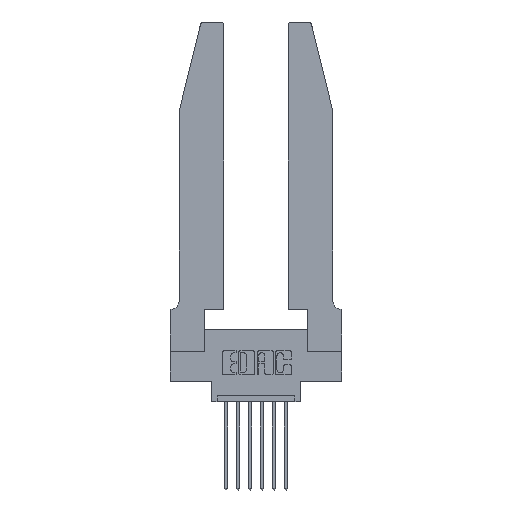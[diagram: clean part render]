
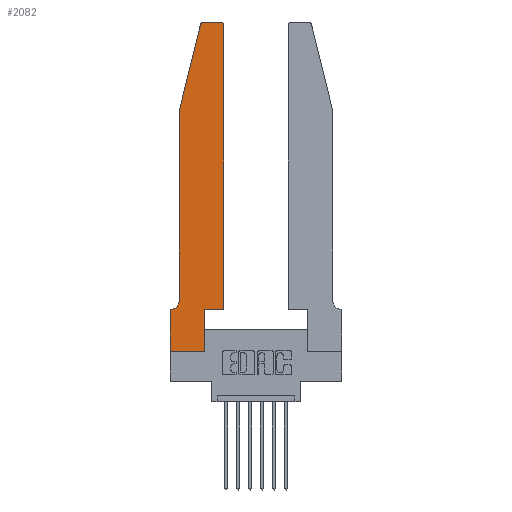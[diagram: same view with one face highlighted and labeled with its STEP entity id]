
A CAD part, top view. The second image highlights one B-rep face of the part: STEP entity #2082.
In plain terms, the highlighted planar face has unit normal (0, 0, 1).
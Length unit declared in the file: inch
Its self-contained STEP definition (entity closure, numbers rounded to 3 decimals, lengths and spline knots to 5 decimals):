
#66 = VECTOR ( 'NONE', #14003, 39.37008 ) ;
#102 = VECTOR ( 'NONE', #5840, 39.37008 ) ;
#453 = CARTESIAN_POINT ( 'NONE',  ( 0.4505, 0.35, 0.37 ) ) ;
#550 = CARTESIAN_POINT ( 'NONE',  ( 0.4205, 2.72, 0.37 ) ) ;
#649 = CARTESIAN_POINT ( 'NONE',  ( 0.2865, 0.35, 0.37 ) ) ;
#678 = EDGE_CURVE ( 'NONE', #8250, #14021, #8763, .T. ) ;
#988 = VERTEX_POINT ( 'NONE', #13932 ) ;
#1011 = ORIENTED_EDGE ( 'NONE', *, *, #9448, .T. ) ;
#1093 = VECTOR ( 'NONE', #13650, 39.37008 ) ;
#1171 = FACE_OUTER_BOUND ( 'NONE', #6539, .T. ) ;
#1270 = VERTEX_POINT ( 'NONE', #453 ) ;
#1389 = CARTESIAN_POINT ( 'NONE',  ( 0.284, 2.75, 0.37 ) ) ;
#1478 = VECTOR ( 'NONE', #7660, 39.37008 ) ;
#1817 = VERTEX_POINT ( 'NONE', #1389 ) ;
#1842 = VERTEX_POINT ( 'NONE', #7890 ) ;
#1893 = ORIENTED_EDGE ( 'NONE', *, *, #9332, .T. ) ;
#1906 = CARTESIAN_POINT ( 'NONE',  ( 0.0755, 2., 0.37 ) ) ;
#1942 = ORIENTED_EDGE ( 'NONE', *, *, #11887, .T. ) ;
#2082 = ADVANCED_FACE ( 'NONE', ( #1171 ), #2833, .T. ) ;
#2570 = DIRECTION ( 'NONE',  ( 0., 0., 1. ) ) ;
#2833 = PLANE ( 'NONE',  #11426 ) ;
#2865 = VERTEX_POINT ( 'NONE', #6434 ) ;
#2966 = EDGE_CURVE ( 'NONE', #1817, #988, #8417, .T. ) ;
#2976 = DIRECTION ( 'NONE',  ( 0., 0., -1. ) ) ;
#3628 = LINE ( 'NONE', #13742, #13936 ) ;
#3701 = ORIENTED_EDGE ( 'NONE', *, *, #10732, .T. ) ;
#3813 = DIRECTION ( 'NONE',  ( 1., 0., 0. ) ) ;
#3830 = LINE ( 'NONE', #8768, #14129 ) ;
#4001 = ORIENTED_EDGE ( 'NONE', *, *, #5350, .T. ) ;
#4075 = DIRECTION ( 'NONE',  ( -1., 0., 0. ) ) ;
#4324 = DIRECTION ( 'NONE',  ( 0., -1., 0. ) ) ;
#4795 = ORIENTED_EDGE ( 'NONE', *, *, #6961, .T. ) ;
#4895 = CARTESIAN_POINT ( 'NONE',  ( 0.4505, 0.35, 0.37 ) ) ;
#5023 = EDGE_CURVE ( 'NONE', #1842, #1270, #12653, .T. ) ;
#5350 = EDGE_CURVE ( 'NONE', #13321, #1817, #8893, .T. ) ;
#5401 = ORIENTED_EDGE ( 'NONE', *, *, #2966, .T. ) ;
#5441 = VERTEX_POINT ( 'NONE', #9337 ) ;
#5596 = VERTEX_POINT ( 'NONE', #7854 ) ;
#5840 = DIRECTION ( 'NONE',  ( -1., 0., 0. ) ) ;
#5863 = VECTOR ( 'NONE', #7314, 39.37008 ) ;
#6434 = CARTESIAN_POINT ( 'NONE',  ( 0., 0.35, 0.37 ) ) ;
#6539 = EDGE_LOOP ( 'NONE', ( #4001, #5401, #1942, #6580, #11002, #10204, #3701, #7214, #1011, #8343, #4795, #1893 ) ) ;
#6580 = ORIENTED_EDGE ( 'NONE', *, *, #678, .T. ) ;
#6613 = DIRECTION ( 'NONE',  ( 0., 1., 0. ) ) ;
#6961 = EDGE_CURVE ( 'NONE', #1270, #5596, #3830, .T. ) ;
#7214 = ORIENTED_EDGE ( 'NONE', *, *, #7489, .T. ) ;
#7291 = AXIS2_PLACEMENT_3D ( 'NONE', #9358, #11533, #8386 ) ;
#7314 = DIRECTION ( 'NONE',  ( 0., 1., 0. ) ) ;
#7489 = EDGE_CURVE ( 'NONE', #5441, #11415, #3628, .T. ) ;
#7660 = DIRECTION ( 'NONE',  ( 0., -1., 0. ) ) ;
#7854 = CARTESIAN_POINT ( 'NONE',  ( 0.4505, 2.72, 0.37 ) ) ;
#7890 = CARTESIAN_POINT ( 'NONE',  ( 0.2865, 0.35, 0.37 ) ) ;
#7938 = CIRCLE ( 'NONE', #13310, 0.07 ) ;
#7983 = CARTESIAN_POINT ( 'NONE',  ( 0.4205, 2.75, 0.37 ) ) ;
#8250 = VERTEX_POINT ( 'NONE', #10523 ) ;
#8343 = ORIENTED_EDGE ( 'NONE', *, *, #5023, .T. ) ;
#8351 = EDGE_CURVE ( 'NONE', #14021, #10306, #7938, .T. ) ;
#8386 = DIRECTION ( 'NONE',  ( 1., 0., 0. ) ) ;
#8417 = CIRCLE ( 'NONE', #7291, 0.03 ) ;
#8763 = LINE ( 'NONE', #9825, #11310 ) ;
#8768 = CARTESIAN_POINT ( 'NONE',  ( 0.4505, 0.35, 0.37 ) ) ;
#8779 = LINE ( 'NONE', #14285, #1478 ) ;
#8893 = LINE ( 'NONE', #9677, #11265 ) ;
#9332 = EDGE_CURVE ( 'NONE', #5596, #13321, #12201, .T. ) ;
#9337 = CARTESIAN_POINT ( 'NONE',  ( 0., 0., 0.37 ) ) ;
#9358 = CARTESIAN_POINT ( 'NONE',  ( 0.284, 2.72, 0.37 ) ) ;
#9448 = EDGE_CURVE ( 'NONE', #11415, #1842, #13917, .T. ) ;
#9677 = CARTESIAN_POINT ( 'NONE',  ( 0.2605, 2.75, 0.37 ) ) ;
#9793 = LINE ( 'NONE', #13311, #102 ) ;
#9825 = CARTESIAN_POINT ( 'NONE',  ( 0.0755, 2., 0.37 ) ) ;
#10204 = ORIENTED_EDGE ( 'NONE', *, *, #10894, .T. ) ;
#10306 = VERTEX_POINT ( 'NONE', #13378 ) ;
#10494 = DIRECTION ( 'NONE',  ( 1., 0., 0. ) ) ;
#10516 = CARTESIAN_POINT ( 'NONE',  ( 0., 0.35, 0.37 ) ) ;
#10523 = CARTESIAN_POINT ( 'NONE',  ( 0.0755, 2., 0.37 ) ) ;
#10732 = EDGE_CURVE ( 'NONE', #2865, #5441, #8779, .T. ) ;
#10894 = EDGE_CURVE ( 'NONE', #10306, #2865, #9793, .T. ) ;
#11002 = ORIENTED_EDGE ( 'NONE', *, *, #8351, .T. ) ;
#11016 = CARTESIAN_POINT ( 'NONE',  ( 0.2865, 0., 0.37 ) ) ;
#11228 = AXIS2_PLACEMENT_3D ( 'NONE', #550, #2570, #10494 ) ;
#11265 = VECTOR ( 'NONE', #4075, 39.37008 ) ;
#11310 = VECTOR ( 'NONE', #4324, 39.37008 ) ;
#11415 = VERTEX_POINT ( 'NONE', #11016 ) ;
#11426 = AXIS2_PLACEMENT_3D ( 'NONE', #10516, #11647, #11731 ) ;
#11533 = DIRECTION ( 'NONE',  ( 0., 0., 1. ) ) ;
#11647 = DIRECTION ( 'NONE',  ( 0., 0., 1. ) ) ;
#11731 = DIRECTION ( 'NONE',  ( 1., 0., 0. ) ) ;
#11743 = CARTESIAN_POINT ( 'NONE',  ( 0.0055, 0.42, 0.37 ) ) ;
#11887 = EDGE_CURVE ( 'NONE', #988, #8250, #13666, .T. ) ;
#12201 = CIRCLE ( 'NONE', #11228, 0.03 ) ;
#12399 = CARTESIAN_POINT ( 'NONE',  ( 0.0755, 0.42, 0.37 ) ) ;
#12653 = LINE ( 'NONE', #4895, #1093 ) ;
#13310 = AXIS2_PLACEMENT_3D ( 'NONE', #11743, #2976, #14006 ) ;
#13311 = CARTESIAN_POINT ( 'NONE',  ( 0.0755, 0.35, 0.37 ) ) ;
#13321 = VERTEX_POINT ( 'NONE', #7983 ) ;
#13378 = CARTESIAN_POINT ( 'NONE',  ( 0.0055, 0.35, 0.37 ) ) ;
#13650 = DIRECTION ( 'NONE',  ( 1., 0., 0. ) ) ;
#13666 = LINE ( 'NONE', #1906, #66 ) ;
#13742 = CARTESIAN_POINT ( 'NONE',  ( 0., 0., 0.37 ) ) ;
#13917 = LINE ( 'NONE', #649, #5863 ) ;
#13932 = CARTESIAN_POINT ( 'NONE',  ( 0.25487, 2.72718, 0.37 ) ) ;
#13936 = VECTOR ( 'NONE', #3813, 39.37008 ) ;
#14003 = DIRECTION ( 'NONE',  ( -0.239, -0.971, 0. ) ) ;
#14006 = DIRECTION ( 'NONE',  ( -1., 0., 0. ) ) ;
#14021 = VERTEX_POINT ( 'NONE', #12399 ) ;
#14129 = VECTOR ( 'NONE', #6613, 39.37008 ) ;
#14285 = CARTESIAN_POINT ( 'NONE',  ( 0., 0., 0.37 ) ) ;
